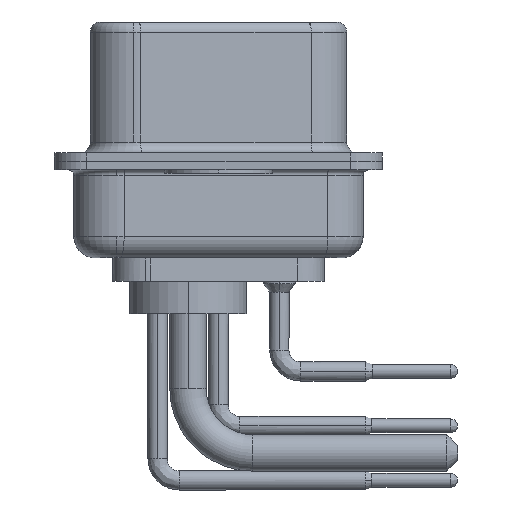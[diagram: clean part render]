
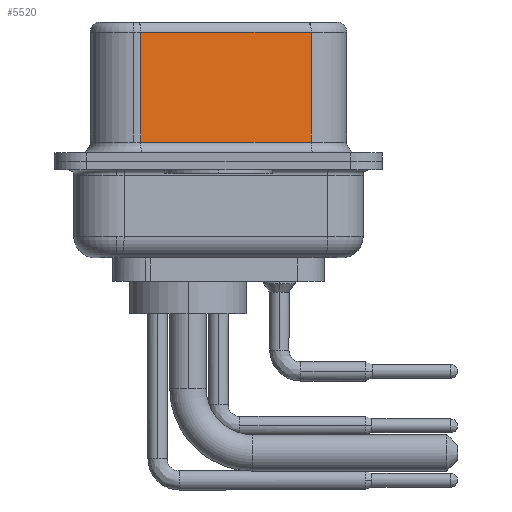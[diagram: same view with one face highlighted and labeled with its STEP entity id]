
A CAD part, left-side view. The second image highlights one B-rep face of the part: STEP entity #5520.
In plain terms, the highlighted planar face has unit normal (-0.985, -0.174, 0).
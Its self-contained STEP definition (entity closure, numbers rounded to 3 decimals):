
#162 = LINE ( 'NONE', #10178, #27091 ) ;
#476 = CARTESIAN_POINT ( 'NONE',  ( 5.132, -4.322, 6.02 ) ) ;
#2359 = VERTEX_POINT ( 'NONE', #31583 ) ;
#2548 = DIRECTION ( 'NONE',  ( 0., 0., -1. ) ) ;
#2867 = CARTESIAN_POINT ( 'NONE',  ( 3.73, 3.628, 6.52 ) ) ;
#3261 = DIRECTION ( 'NONE',  ( 0.174, -0.985, 0. ) ) ;
#3938 = CARTESIAN_POINT ( 'NONE',  ( 5.132, -4.322, 6.02 ) ) ;
#4986 = EDGE_LOOP ( 'NONE', ( #30793, #16562, #18349, #19630 ) ) ;
#5299 = VECTOR ( 'NONE', #2548, 1000. ) ;
#5520 = ADVANCED_FACE ( 'NONE', ( #16446 ), #28910, .F. ) ;
#5552 = LINE ( 'NONE', #15563, #9633 ) ;
#7479 = LINE ( 'NONE', #2867, #5299 ) ;
#8728 = EDGE_CURVE ( 'NONE', #2359, #13006, #5552, .T. ) ;
#8930 = AXIS2_PLACEMENT_3D ( 'NONE', #13820, #26116, #13990 ) ;
#9633 = VECTOR ( 'NONE', #3261, 1000. ) ;
#10178 = CARTESIAN_POINT ( 'NONE',  ( 5.132, -4.322, 6.52 ) ) ;
#13006 = VERTEX_POINT ( 'NONE', #22226 ) ;
#13820 = CARTESIAN_POINT ( 'NONE',  ( 5.132, -4.322, 6.52 ) ) ;
#13990 = DIRECTION ( 'NONE',  ( -0.174, 0.985, 0. ) ) ;
#15563 = CARTESIAN_POINT ( 'NONE',  ( 5.132, -4.322, 0.9 ) ) ;
#15762 = EDGE_CURVE ( 'NONE', #25335, #22428, #19807, .T. ) ;
#16446 = FACE_OUTER_BOUND ( 'NONE', #4986, .T. ) ;
#16562 = ORIENTED_EDGE ( 'NONE', *, *, #15762, .T. ) ;
#17209 = EDGE_CURVE ( 'NONE', #25335, #13006, #162, .T. ) ;
#18349 = ORIENTED_EDGE ( 'NONE', *, *, #32290, .T. ) ;
#19630 = ORIENTED_EDGE ( 'NONE', *, *, #8728, .T. ) ;
#19807 = LINE ( 'NONE', #476, #20743 ) ;
#20154 = DIRECTION ( 'NONE',  ( 0., 0., -1. ) ) ;
#20743 = VECTOR ( 'NONE', #25377, 1000. ) ;
#21180 = CARTESIAN_POINT ( 'NONE',  ( 3.73, 3.628, 6.02 ) ) ;
#22226 = CARTESIAN_POINT ( 'NONE',  ( 5.132, -4.322, 0.9 ) ) ;
#22428 = VERTEX_POINT ( 'NONE', #21180 ) ;
#25335 = VERTEX_POINT ( 'NONE', #3938 ) ;
#25377 = DIRECTION ( 'NONE',  ( -0.174, 0.985, 0. ) ) ;
#26116 = DIRECTION ( 'NONE',  ( 0.985, 0.174, 0. ) ) ;
#27091 = VECTOR ( 'NONE', #20154, 1000. ) ;
#28910 = PLANE ( 'NONE',  #8930 ) ;
#30793 = ORIENTED_EDGE ( 'NONE', *, *, #17209, .F. ) ;
#31583 = CARTESIAN_POINT ( 'NONE',  ( 3.73, 3.628, 0.9 ) ) ;
#32290 = EDGE_CURVE ( 'NONE', #22428, #2359, #7479, .T. ) ;
